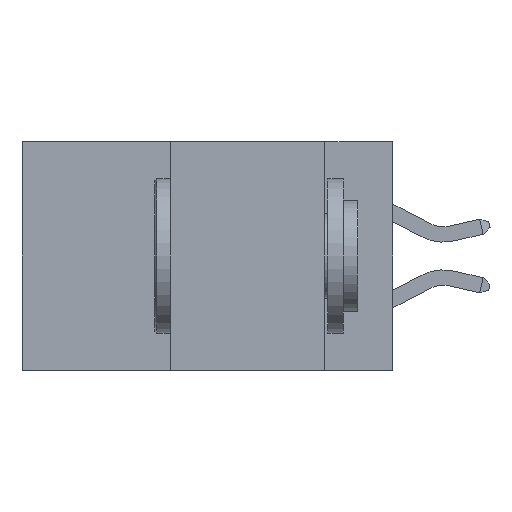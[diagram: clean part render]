
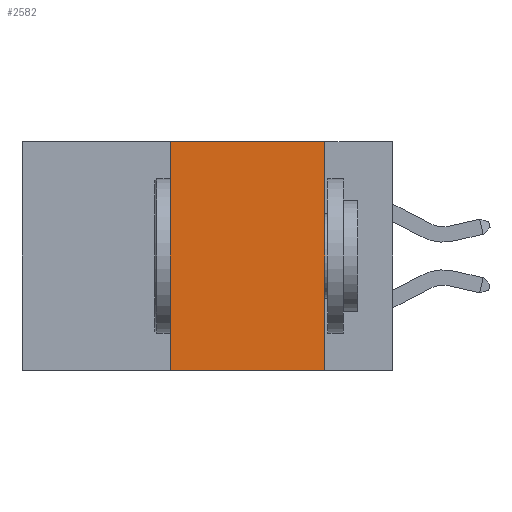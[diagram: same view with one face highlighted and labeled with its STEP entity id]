
A CAD part, left-side view. The second image highlights one B-rep face of the part: STEP entity #2582.
In plain terms, the highlighted planar face has unit normal (-1, 0, 0).
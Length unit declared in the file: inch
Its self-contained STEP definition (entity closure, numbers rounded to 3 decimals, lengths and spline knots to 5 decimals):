
#133 = VECTOR ( 'NONE', #9233, 39.37008 ) ;
#580 = CARTESIAN_POINT ( 'NONE',  ( 0., 0.36, 0. ) ) ;
#1367 = CARTESIAN_POINT ( 'NONE',  ( 0., 0.36, 0. ) ) ;
#1968 = CARTESIAN_POINT ( 'NONE',  ( 0., 0.11, 0. ) ) ;
#2456 = DIRECTION ( 'NONE',  ( 0., 0., -1. ) ) ;
#2582 = ADVANCED_FACE ( 'NONE', ( #13947 ), #17576, .F. ) ;
#3326 = CARTESIAN_POINT ( 'NONE',  ( 0., 0.6, -0.37 ) ) ;
#3555 = ORIENTED_EDGE ( 'NONE', *, *, #7585, .T. ) ;
#4906 = LINE ( 'NONE', #580, #9158 ) ;
#5066 = LINE ( 'NONE', #7895, #133 ) ;
#5434 = ORIENTED_EDGE ( 'NONE', *, *, #8489, .F. ) ;
#5524 = VERTEX_POINT ( 'NONE', #14114 ) ;
#5525 = ORIENTED_EDGE ( 'NONE', *, *, #8436, .F. ) ;
#6039 = EDGE_CURVE ( 'NONE', #15308, #17076, #5066, .T. ) ;
#6179 = EDGE_LOOP ( 'NONE', ( #5525, #10459, #5434, #3555 ) ) ;
#7437 = LINE ( 'NONE', #1968, #13644 ) ;
#7550 = CARTESIAN_POINT ( 'NONE',  ( 0., 0.11, 0. ) ) ;
#7585 = EDGE_CURVE ( 'NONE', #5524, #9413, #8225, .T. ) ;
#7895 = CARTESIAN_POINT ( 'NONE',  ( 0., 0.6, 0. ) ) ;
#8225 = LINE ( 'NONE', #3326, #15944 ) ;
#8436 = EDGE_CURVE ( 'NONE', #17076, #9413, #7437, .T. ) ;
#8489 = EDGE_CURVE ( 'NONE', #5524, #15308, #4906, .T. ) ;
#8909 = AXIS2_PLACEMENT_3D ( 'NONE', #12066, #9385, #2456 ) ;
#9158 = VECTOR ( 'NONE', #15989, 39.37008 ) ;
#9233 = DIRECTION ( 'NONE',  ( 0., -1., 0. ) ) ;
#9385 = DIRECTION ( 'NONE',  ( 1., 0., 0. ) ) ;
#9413 = VERTEX_POINT ( 'NONE', #15745 ) ;
#10459 = ORIENTED_EDGE ( 'NONE', *, *, #6039, .F. ) ;
#12066 = CARTESIAN_POINT ( 'NONE',  ( 0., 0.6, 0. ) ) ;
#13644 = VECTOR ( 'NONE', #17017, 39.37008 ) ;
#13947 = FACE_OUTER_BOUND ( 'NONE', #6179, .T. ) ;
#14114 = CARTESIAN_POINT ( 'NONE',  ( 0., 0.36, -0.37 ) ) ;
#14286 = DIRECTION ( 'NONE',  ( 0., -1., 0. ) ) ;
#15308 = VERTEX_POINT ( 'NONE', #1367 ) ;
#15745 = CARTESIAN_POINT ( 'NONE',  ( 0., 0.11, -0.37 ) ) ;
#15944 = VECTOR ( 'NONE', #14286, 39.37008 ) ;
#15989 = DIRECTION ( 'NONE',  ( 0., 0., 1. ) ) ;
#17017 = DIRECTION ( 'NONE',  ( 0., 0., -1. ) ) ;
#17076 = VERTEX_POINT ( 'NONE', #7550 ) ;
#17576 = PLANE ( 'NONE',  #8909 ) ;
